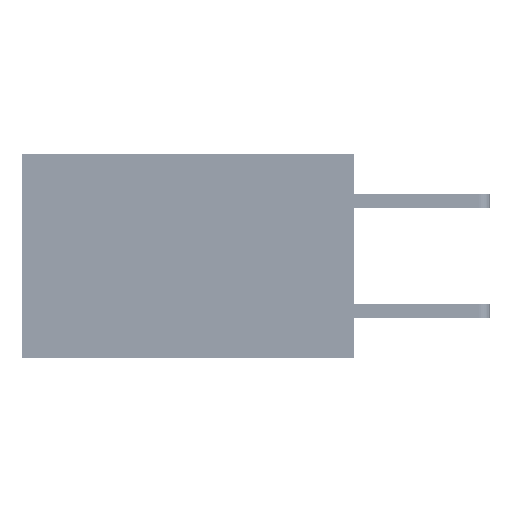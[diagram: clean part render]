
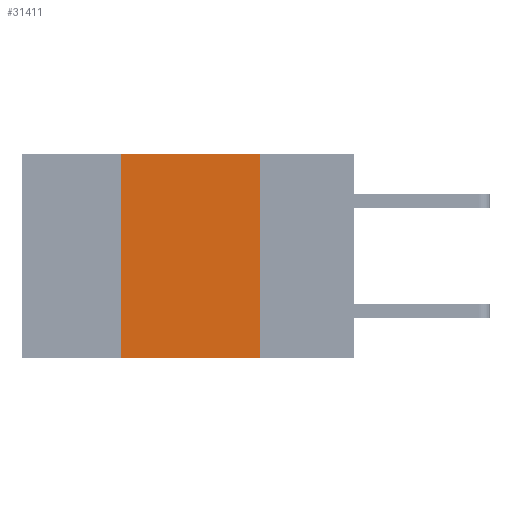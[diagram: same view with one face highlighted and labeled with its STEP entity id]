
A CAD part, left-side view. The second image highlights one B-rep face of the part: STEP entity #31411.
In plain terms, the highlighted planar face has unit normal (-1, 0, 0).
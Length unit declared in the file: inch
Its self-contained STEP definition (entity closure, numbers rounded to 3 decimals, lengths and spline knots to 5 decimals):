
#462 = CARTESIAN_POINT ( 'NONE',  ( 0., 0.6, 0. ) ) ;
#1311 = CARTESIAN_POINT ( 'NONE',  ( 0., 0.42, -0.37 ) ) ;
#2026 = VERTEX_POINT ( 'NONE', #1311 ) ;
#2816 = CARTESIAN_POINT ( 'NONE',  ( 0., 0.42, 0. ) ) ;
#2863 = DIRECTION ( 'NONE',  ( 1., 0., 0. ) ) ;
#3655 = EDGE_CURVE ( 'NONE', #8191, #14095, #29678, .T. ) ;
#3792 = DIRECTION ( 'NONE',  ( 0., -1., 0. ) ) ;
#4197 = VERTEX_POINT ( 'NONE', #2816 ) ;
#5111 = CARTESIAN_POINT ( 'NONE',  ( 0., 0.17, 0. ) ) ;
#5347 = ORIENTED_EDGE ( 'NONE', *, *, #3655, .F. ) ;
#6581 = CARTESIAN_POINT ( 'NONE',  ( 0., 0.17, 0. ) ) ;
#7589 = LINE ( 'NONE', #18655, #24421 ) ;
#8191 = VERTEX_POINT ( 'NONE', #5111 ) ;
#10156 = CARTESIAN_POINT ( 'NONE',  ( 0., 0.6, -0.37 ) ) ;
#10598 = AXIS2_PLACEMENT_3D ( 'NONE', #40613, #2863, #24976 ) ;
#11177 = VECTOR ( 'NONE', #35465, 39.37008 ) ;
#14095 = VERTEX_POINT ( 'NONE', #38871 ) ;
#14231 = ORIENTED_EDGE ( 'NONE', *, *, #33617, .T. ) ;
#14691 = EDGE_CURVE ( 'NONE', #4197, #8191, #23508, .T. ) ;
#15078 = VECTOR ( 'NONE', #3792, 39.37008 ) ;
#18604 = PLANE ( 'NONE',  #10598 ) ;
#18655 = CARTESIAN_POINT ( 'NONE',  ( 0., 0.42, 0. ) ) ;
#22612 = DIRECTION ( 'NONE',  ( 0., 0., -1. ) ) ;
#22734 = FACE_OUTER_BOUND ( 'NONE', #24649, .T. ) ;
#23040 = EDGE_CURVE ( 'NONE', #2026, #4197, #7589, .T. ) ;
#23508 = LINE ( 'NONE', #462, #15078 ) ;
#23682 = ORIENTED_EDGE ( 'NONE', *, *, #14691, .F. ) ;
#24421 = VECTOR ( 'NONE', #25033, 39.37008 ) ;
#24649 = EDGE_LOOP ( 'NONE', ( #5347, #23682, #28606, #14231 ) ) ;
#24976 = DIRECTION ( 'NONE',  ( 0., 0., -1. ) ) ;
#25033 = DIRECTION ( 'NONE',  ( 0., 0., 1. ) ) ;
#27993 = LINE ( 'NONE', #10156, #11177 ) ;
#28606 = ORIENTED_EDGE ( 'NONE', *, *, #23040, .F. ) ;
#29678 = LINE ( 'NONE', #6581, #38024 ) ;
#31411 = ADVANCED_FACE ( 'NONE', ( #22734 ), #18604, .F. ) ;
#33617 = EDGE_CURVE ( 'NONE', #2026, #14095, #27993, .T. ) ;
#35465 = DIRECTION ( 'NONE',  ( 0., -1., 0. ) ) ;
#38024 = VECTOR ( 'NONE', #22612, 39.37008 ) ;
#38871 = CARTESIAN_POINT ( 'NONE',  ( 0., 0.17, -0.37 ) ) ;
#40613 = CARTESIAN_POINT ( 'NONE',  ( 0., 0.6, 0. ) ) ;
